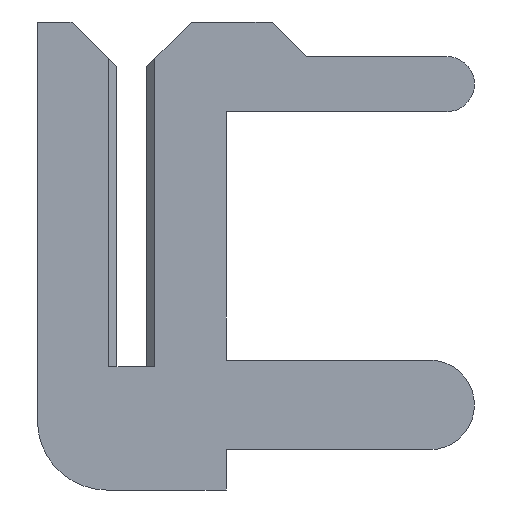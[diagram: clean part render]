
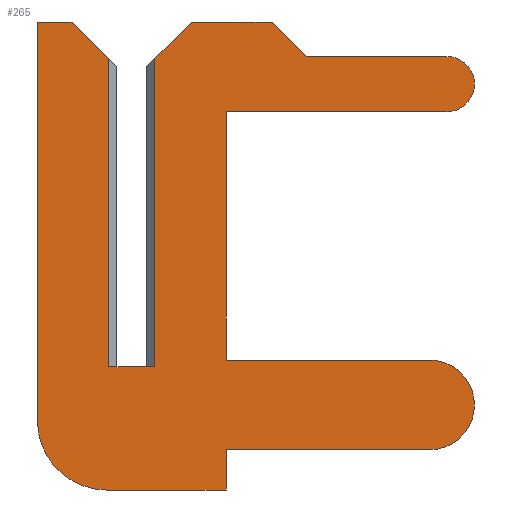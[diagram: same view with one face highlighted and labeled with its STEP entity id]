
A CAD part, left-side view. The second image highlights one B-rep face of the part: STEP entity #265.
In plain terms, the highlighted planar face has unit normal (-1, 0, 0).
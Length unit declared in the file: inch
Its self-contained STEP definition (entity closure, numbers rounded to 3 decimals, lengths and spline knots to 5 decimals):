
#1 = DIRECTION ( 'NONE',  ( 0., 0., 1. ) ) ;
#2 = EDGE_CURVE ( 'NONE', #120, #1247, #933, .T. ) ;
#20 = DIRECTION ( 'NONE',  ( 0., -0.707, 0.707 ) ) ;
#36 = VERTEX_POINT ( 'NONE', #623 ) ;
#37 = ORIENTED_EDGE ( 'NONE', *, *, #889, .F. ) ;
#55 = ORIENTED_EDGE ( 'NONE', *, *, #146, .F. ) ;
#58 = CARTESIAN_POINT ( 'NONE',  ( -0.01, -0.137, 0.123 ) ) ;
#62 = VECTOR ( 'NONE', #827, 39.37008 ) ;
#79 = CARTESIAN_POINT ( 'NONE',  ( -0.01, -0.137, 0.135 ) ) ;
#84 = ORIENTED_EDGE ( 'NONE', *, *, #729, .T. ) ;
#90 = EDGE_CURVE ( 'NONE', #164, #804, #747, .T. ) ;
#100 = LINE ( 'NONE', #901, #807 ) ;
#104 = DIRECTION ( 'NONE',  ( 0., -0.707, -0.707 ) ) ;
#105 = ORIENTED_EDGE ( 'NONE', *, *, #1017, .F. ) ;
#113 = CARTESIAN_POINT ( 'NONE',  ( -0.01, 0.026, 0.15 ) ) ;
#114 = CARTESIAN_POINT ( 'NONE',  ( -0.01, -0.01, 0.15 ) ) ;
#117 = CARTESIAN_POINT ( 'NONE',  ( -0.01, -0.041, -0.036 ) ) ;
#120 = VERTEX_POINT ( 'NONE', #538 ) ;
#126 = VERTEX_POINT ( 'NONE', #1027 ) ;
#133 = DIRECTION ( 'NONE',  ( 0., 0., -1. ) ) ;
#140 = DIRECTION ( 'NONE',  ( 0., -0.707, -0.707 ) ) ;
#146 = EDGE_CURVE ( 'NONE', #1247, #732, #609, .T. ) ;
#147 = CARTESIAN_POINT ( 'NONE',  ( -0.01, 0.011, -0.0535 ) ) ;
#151 = VERTEX_POINT ( 'NONE', #1138 ) ;
#162 = EDGE_CURVE ( 'NONE', #1070, #323, #874, .T. ) ;
#164 = VERTEX_POINT ( 'NONE', #236 ) ;
#195 = CARTESIAN_POINT ( 'NONE',  ( -0.01, 0.0065, 0. ) ) ;
#204 = CARTESIAN_POINT ( 'NONE',  ( -0.01, -0.041, 0.111 ) ) ;
#215 = DIRECTION ( 'NONE',  ( 0., 1., 0. ) ) ;
#218 = ORIENTED_EDGE ( 'NONE', *, *, #279, .F. ) ;
#228 = CIRCLE ( 'NONE', #1154, 0.03 ) ;
#236 = CARTESIAN_POINT ( 'NONE',  ( -0.01, 0.041, 0.15 ) ) ;
#237 = DIRECTION ( 'NONE',  ( 0., 0., 1. ) ) ;
#238 = ORIENTED_EDGE ( 'NONE', *, *, #294, .F. ) ;
#249 = VECTOR ( 'NONE', #215, 39.37008 ) ;
#265 = ADVANCED_FACE ( 'NONE', ( #814 ), #511, .T. ) ;
#271 = CARTESIAN_POINT ( 'NONE',  ( -0.01, 0.026, 0.15 ) ) ;
#279 = EDGE_CURVE ( 'NONE', #126, #1070, #1237, .T. ) ;
#294 = EDGE_CURVE ( 'NONE', #732, #126, #736, .T. ) ;
#299 = CARTESIAN_POINT ( 'NONE',  ( -0.01, -0.1295, 0.003 ) ) ;
#313 = DIRECTION ( 'NONE',  ( 0., 0., 1. ) ) ;
#323 = VERTEX_POINT ( 'NONE', #117 ) ;
#332 = ORIENTED_EDGE ( 'NONE', *, *, #481, .F. ) ;
#337 = CARTESIAN_POINT ( 'NONE',  ( -0.01, -0.041, 0.003 ) ) ;
#384 = EDGE_CURVE ( 'NONE', #323, #36, #440, .T. ) ;
#390 = CARTESIAN_POINT ( 'NONE',  ( -0.01, -0.076, 0.135 ) ) ;
#409 = CARTESIAN_POINT ( 'NONE',  ( -0.01, -0.1295, -0.036 ) ) ;
#412 = DIRECTION ( 'NONE',  ( 0., 0., -1. ) ) ;
#413 = ORIENTED_EDGE ( 'NONE', *, *, #921, .F. ) ;
#431 = VERTEX_POINT ( 'NONE', #718 ) ;
#440 = LINE ( 'NONE', #1112, #1093 ) ;
#446 = CARTESIAN_POINT ( 'NONE',  ( -0.01, -0.01, 0.134 ) ) ;
#472 = DIRECTION ( 'NONE',  ( 0., 0., 1. ) ) ;
#481 = EDGE_CURVE ( 'NONE', #513, #951, #880, .T. ) ;
#483 = CARTESIAN_POINT ( 'NONE',  ( -0.01, 0.01, -0.0235 ) ) ;
#506 = DIRECTION ( 'NONE',  ( 0., -1., 0. ) ) ;
#509 = CARTESIAN_POINT ( 'NONE',  ( -0.01, -0.026, 0.15 ) ) ;
#511 = PLANE ( 'NONE',  #1182 ) ;
#513 = VERTEX_POINT ( 'NONE', #1019 ) ;
#517 = CARTESIAN_POINT ( 'NONE',  ( -0.01, -0.1295, -0.0165 ) ) ;
#519 = DIRECTION ( 'NONE',  ( 0., 0., 1. ) ) ;
#524 = VECTOR ( 'NONE', #812, 39.37008 ) ;
#525 = VECTOR ( 'NONE', #104, 39.37008 ) ;
#538 = CARTESIAN_POINT ( 'NONE',  ( -0.01, -0.137, 0.111 ) ) ;
#546 = CARTESIAN_POINT ( 'NONE',  ( -0.01, 0.011, -0.0535 ) ) ;
#579 = EDGE_CURVE ( 'NONE', #1240, #120, #728, .T. ) ;
#585 = DIRECTION ( 'NONE',  ( 1., 0., 0. ) ) ;
#593 = CARTESIAN_POINT ( 'NONE',  ( -0.01, 0.0065, 0.1305 ) ) ;
#609 = LINE ( 'NONE', #337, #723 ) ;
#615 = ORIENTED_EDGE ( 'NONE', *, *, #946, .F. ) ;
#623 = CARTESIAN_POINT ( 'NONE',  ( -0.01, -0.041, -0.0535 ) ) ;
#637 = VERTEX_POINT ( 'NONE', #759 ) ;
#647 = ORIENTED_EDGE ( 'NONE', *, *, #1193, .F. ) ;
#651 = VERTEX_POINT ( 'NONE', #546 ) ;
#668 = VERTEX_POINT ( 'NONE', #446 ) ;
#670 = ORIENTED_EDGE ( 'NONE', *, *, #2, .F. ) ;
#680 = LINE ( 'NONE', #719, #865 ) ;
#698 = DIRECTION ( 'NONE',  ( 0., 0., 1. ) ) ;
#714 = DIRECTION ( 'NONE',  ( 1., 0., 0. ) ) ;
#718 = CARTESIAN_POINT ( 'NONE',  ( -0.01, 0.01, 0.134 ) ) ;
#719 = CARTESIAN_POINT ( 'NONE',  ( -0.01, 0.041, 0.15 ) ) ;
#723 = VECTOR ( 'NONE', #133, 39.37008 ) ;
#728 = CIRCLE ( 'NONE', #1045, 0.012 ) ;
#729 = EDGE_CURVE ( 'NONE', #637, #431, #774, .T. ) ;
#732 = VERTEX_POINT ( 'NONE', #1276 ) ;
#736 = LINE ( 'NONE', #299, #922 ) ;
#737 = CARTESIAN_POINT ( 'NONE',  ( -0.01, -0.041, -0.036 ) ) ;
#747 = LINE ( 'NONE', #113, #62 ) ;
#758 = VECTOR ( 'NONE', #1191, 39.37008 ) ;
#759 = CARTESIAN_POINT ( 'NONE',  ( -0.01, 0.01, 0. ) ) ;
#767 = CARTESIAN_POINT ( 'NONE',  ( -0.01, -0.026, 0.15 ) ) ;
#774 = LINE ( 'NONE', #483, #1274 ) ;
#788 = ORIENTED_EDGE ( 'NONE', *, *, #90, .F. ) ;
#795 = ORIENTED_EDGE ( 'NONE', *, *, #384, .F. ) ;
#804 = VERTEX_POINT ( 'NONE', #271 ) ;
#807 = VECTOR ( 'NONE', #20, 39.37008 ) ;
#812 = DIRECTION ( 'NONE',  ( 0., 0., -1. ) ) ;
#814 = FACE_OUTER_BOUND ( 'NONE', #1149, .T. ) ;
#818 = DIRECTION ( 'NONE',  ( -1., 0., 0. ) ) ;
#823 = VECTOR ( 'NONE', #1040, 39.37008 ) ;
#827 = DIRECTION ( 'NONE',  ( 0., -1., 0. ) ) ;
#838 = DIRECTION ( 'NONE',  ( 0., 1., 0. ) ) ;
#850 = LINE ( 'NONE', #1016, #1270 ) ;
#865 = VECTOR ( 'NONE', #313, 39.37008 ) ;
#873 = EDGE_CURVE ( 'NONE', #804, #431, #1056, .T. ) ;
#874 = LINE ( 'NONE', #737, #1111 ) ;
#880 = LINE ( 'NONE', #916, #927 ) ;
#889 = EDGE_CURVE ( 'NONE', #989, #513, #1025, .T. ) ;
#901 = CARTESIAN_POINT ( 'NONE',  ( -0.01, -0.0065, 0.1305 ) ) ;
#910 = ORIENTED_EDGE ( 'NONE', *, *, #162, .F. ) ;
#911 = LINE ( 'NONE', #147, #823 ) ;
#916 = CARTESIAN_POINT ( 'NONE',  ( -0.01, -0.076, 0.135 ) ) ;
#921 = EDGE_CURVE ( 'NONE', #651, #1131, #228, .T. ) ;
#922 = VECTOR ( 'NONE', #506, 39.37008 ) ;
#927 = VECTOR ( 'NONE', #140, 39.37008 ) ;
#933 = LINE ( 'NONE', #204, #249 ) ;
#946 = EDGE_CURVE ( 'NONE', #637, #151, #1257, .T. ) ;
#951 = VERTEX_POINT ( 'NONE', #390 ) ;
#975 = CARTESIAN_POINT ( 'NONE',  ( -0.01, -0.041, 0.111 ) ) ;
#989 = VERTEX_POINT ( 'NONE', #509 ) ;
#991 = VECTOR ( 'NONE', #1185, 39.37008 ) ;
#995 = EDGE_CURVE ( 'NONE', #668, #989, #100, .T. ) ;
#998 = ORIENTED_EDGE ( 'NONE', *, *, #995, .F. ) ;
#1016 = CARTESIAN_POINT ( 'NONE',  ( -0.01, -0.137, 0.135 ) ) ;
#1017 = EDGE_CURVE ( 'NONE', #1131, #164, #680, .T. ) ;
#1019 = CARTESIAN_POINT ( 'NONE',  ( -0.01, -0.061, 0.15 ) ) ;
#1025 = LINE ( 'NONE', #767, #758 ) ;
#1027 = CARTESIAN_POINT ( 'NONE',  ( -0.01, -0.1295, 0.003 ) ) ;
#1040 = DIRECTION ( 'NONE',  ( 0., 1., 0. ) ) ;
#1045 = AXIS2_PLACEMENT_3D ( 'NONE', #58, #1239, #237 ) ;
#1055 = ORIENTED_EDGE ( 'NONE', *, *, #579, .F. ) ;
#1056 = LINE ( 'NONE', #593, #525 ) ;
#1067 = ORIENTED_EDGE ( 'NONE', *, *, #873, .F. ) ;
#1070 = VERTEX_POINT ( 'NONE', #409 ) ;
#1075 = EDGE_CURVE ( 'NONE', #668, #151, #1162, .T. ) ;
#1081 = ORIENTED_EDGE ( 'NONE', *, *, #1094, .F. ) ;
#1093 = VECTOR ( 'NONE', #412, 39.37008 ) ;
#1094 = EDGE_CURVE ( 'NONE', #951, #1240, #850, .T. ) ;
#1109 = DIRECTION ( 'NONE',  ( 0., -1., 0. ) ) ;
#1111 = VECTOR ( 'NONE', #838, 39.37008 ) ;
#1112 = CARTESIAN_POINT ( 'NONE',  ( -0.01, -0.041, -0.0535 ) ) ;
#1123 = AXIS2_PLACEMENT_3D ( 'NONE', #517, #714, #1 ) ;
#1131 = VERTEX_POINT ( 'NONE', #1238 ) ;
#1138 = CARTESIAN_POINT ( 'NONE',  ( -0.01, -0.01, 0. ) ) ;
#1149 = EDGE_LOOP ( 'NONE', ( #998, #1255, #615, #84, #1067, #788, #105, #413, #647, #795, #910, #218, #238, #55, #670, #1055, #1081, #332, #37 ) ) ;
#1154 = AXIS2_PLACEMENT_3D ( 'NONE', #1179, #585, #519 ) ;
#1162 = LINE ( 'NONE', #114, #524 ) ;
#1179 = CARTESIAN_POINT ( 'NONE',  ( -0.01, 0.011, -0.0235 ) ) ;
#1182 = AXIS2_PLACEMENT_3D ( 'NONE', #1211, #818, #698 ) ;
#1185 = DIRECTION ( 'NONE',  ( 0., -1., 0. ) ) ;
#1191 = DIRECTION ( 'NONE',  ( 0., -1., 0. ) ) ;
#1193 = EDGE_CURVE ( 'NONE', #36, #651, #911, .T. ) ;
#1211 = CARTESIAN_POINT ( 'NONE',  ( -0.01, 0.011, -0.0235 ) ) ;
#1237 = CIRCLE ( 'NONE', #1123, 0.0195 ) ;
#1238 = CARTESIAN_POINT ( 'NONE',  ( -0.01, 0.041, -0.0235 ) ) ;
#1239 = DIRECTION ( 'NONE',  ( 1., 0., 0. ) ) ;
#1240 = VERTEX_POINT ( 'NONE', #79 ) ;
#1247 = VERTEX_POINT ( 'NONE', #975 ) ;
#1255 = ORIENTED_EDGE ( 'NONE', *, *, #1075, .T. ) ;
#1257 = LINE ( 'NONE', #195, #991 ) ;
#1270 = VECTOR ( 'NONE', #1109, 39.37008 ) ;
#1274 = VECTOR ( 'NONE', #472, 39.37008 ) ;
#1276 = CARTESIAN_POINT ( 'NONE',  ( -0.01, -0.041, 0.003 ) ) ;
